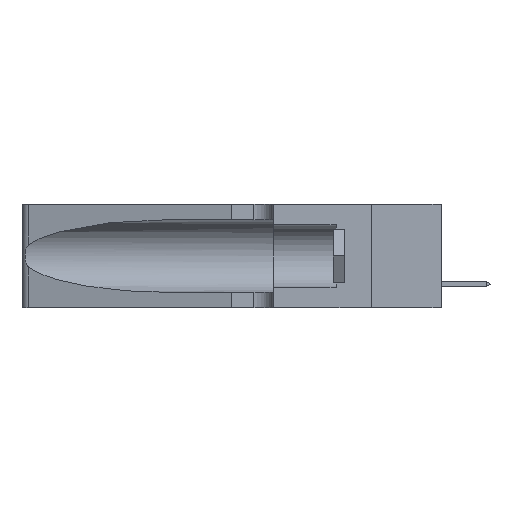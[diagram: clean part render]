
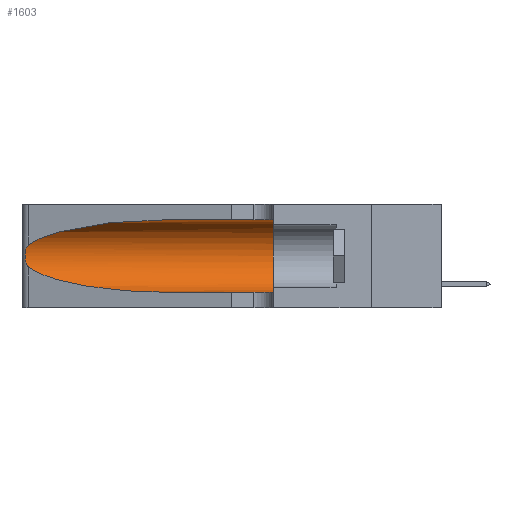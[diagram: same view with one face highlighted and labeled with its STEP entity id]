
A CAD part, left-side view. The second image highlights one B-rep face of the part: STEP entity #1603.
In plain terms, the highlighted cylindrical face has radius 3.308 mm (diameter 6.617 mm), a partial arc.
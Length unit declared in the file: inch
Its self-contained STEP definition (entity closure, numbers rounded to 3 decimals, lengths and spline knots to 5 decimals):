
#150 = AXIS2_PLACEMENT_3D ( 'NONE', #41424, #35982, #982 ) ;
#260 = VERTEX_POINT ( 'NONE', #41802 ) ;
#375 = EDGE_CURVE ( 'NONE', #417, #260, #31418, .T. ) ;
#417 = VERTEX_POINT ( 'NONE', #14140 ) ;
#982 = DIRECTION ( 'NONE',  ( 0., 0., 1. ) ) ;
#1032 = VERTEX_POINT ( 'NONE', #37937 ) ;
#1080 = VERTEX_POINT ( 'NONE', #20702 ) ;
#1603 = ADVANCED_FACE ( 'NONE', ( #44510 ), #25663, .F. ) ;
#2591 = CARTESIAN_POINT ( 'NONE',  ( 0.25555, 1.22993, 0.14849 ) ) ;
#4481 = EDGE_CURVE ( 'NONE', #1080, #30819, #5977, .T. ) ;
#5298 = VECTOR ( 'NONE', #27227, 39.37008 ) ;
#5703 = EDGE_CURVE ( 'NONE', #1080, #417, #10057, .T. ) ;
#5969 = CARTESIAN_POINT ( 'NONE',  ( 0.25487, 1.22718, 0.14631 ) ) ;
#5977 = LINE ( 'NONE', #21402, #46657 ) ;
#6178 = CARTESIAN_POINT ( 'NONE',  ( 0.25487, 1.22718, 0.14631 ) ) ;
#6469 = CARTESIAN_POINT ( 'NONE',  ( 0.25487, 1.22718, 0.22369 ) ) ;
#6504 = CARTESIAN_POINT ( 'NONE',  ( 0.26018, 1.23835, 0.19895 ) ) ;
#9677 = CARTESIAN_POINT ( 'NONE',  ( 0.25639, 1.23184, 0.21858 ) ) ;
#9921 = CIRCLE ( 'NONE', #150, 0.13025 ) ;
#9954 = CARTESIAN_POINT ( 'NONE',  ( 0.1305, 0.72297, 0.05475 ) ) ;
#9999 = CARTESIAN_POINT ( 'NONE',  ( 0.25639, 1.23186, 0.15144 ) ) ;
#10057 =( BOUNDED_CURVE ( )  B_SPLINE_CURVE ( 3, ( #39265, #17660, #21315, #6469 ),
 .UNSPECIFIED., .F., .F. ) 
 B_SPLINE_CURVE_WITH_KNOTS ( ( 4, 4 ),
 ( 1.5708, 2.84003 ),
 .UNSPECIFIED. ) 
 CURVE ( )  GEOMETRIC_REPRESENTATION_ITEM ( )  RATIONAL_B_SPLINE_CURVE ( ( 1., 0.87, 0.87, 1. ) ) 
 REPRESENTATION_ITEM ( '' )  );
#10159 = CARTESIAN_POINT ( 'NONE',  ( 0.26075, 1.23896, 0.178 ) ) ;
#11439 =( BOUNDED_CURVE ( )  B_SPLINE_CURVE ( 3, ( #5969, #35218, #43255, #9954 ),
 .UNSPECIFIED., .F., .F. ) 
 B_SPLINE_CURVE_WITH_KNOTS ( ( 4, 4 ),
 ( 3.44316, 4.71239 ),
 .UNSPECIFIED. ) 
 CURVE ( )  GEOMETRIC_REPRESENTATION_ITEM ( )  RATIONAL_B_SPLINE_CURVE ( ( 1., 0.87, 0.87, 1. ) ) 
 REPRESENTATION_ITEM ( '' )  );
#12462 = EDGE_LOOP ( 'NONE', ( #20390, #26127, #23223, #43813, #46731, #25531 ) ) ;
#13344 = CARTESIAN_POINT ( 'NONE',  ( 0.25854, 1.2359, 0.20912 ) ) ;
#14140 = CARTESIAN_POINT ( 'NONE',  ( 0.25487, 1.22718, 0.22369 ) ) ;
#14780 = EDGE_CURVE ( 'NONE', #31597, #1032, #15014, .T. ) ;
#15014 = LINE ( 'NONE', #30745, #5298 ) ;
#16245 = CARTESIAN_POINT ( 'NONE',  ( 0.1305, 0.72297, 0.05475 ) ) ;
#17043 = CARTESIAN_POINT ( 'NONE',  ( 0.25856, 1.23593, 0.16098 ) ) ;
#17660 = CARTESIAN_POINT ( 'NONE',  ( 0.18966, 0.96281, 0.31525 ) ) ;
#20390 = ORIENTED_EDGE ( 'NONE', *, *, #5703, .T. ) ;
#20414 = EDGE_CURVE ( 'NONE', #30819, #1032, #9921, .T. ) ;
#20702 = CARTESIAN_POINT ( 'NONE',  ( 0.1305, 0.72297, 0.31525 ) ) ;
#21315 = CARTESIAN_POINT ( 'NONE',  ( 0.2373, 1.15595, 0.28018 ) ) ;
#21402 = CARTESIAN_POINT ( 'NONE',  ( 0.1305, 1.61858, 0.31525 ) ) ;
#21856 = DIRECTION ( 'NONE',  ( 0., -1., 0. ) ) ;
#23223 = ORIENTED_EDGE ( 'NONE', *, *, #28506, .T. ) ;
#24023 = CARTESIAN_POINT ( 'NONE',  ( 0.1305, 1.61858, 0.185 ) ) ;
#24521 = CARTESIAN_POINT ( 'NONE',  ( 0.26017, 1.23833, 0.17102 ) ) ;
#25531 = ORIENTED_EDGE ( 'NONE', *, *, #4481, .F. ) ;
#25663 = CYLINDRICAL_SURFACE ( 'NONE', #47308, 0.13025 ) ;
#26127 = ORIENTED_EDGE ( 'NONE', *, *, #375, .T. ) ;
#26892 = CARTESIAN_POINT ( 'NONE',  ( 0.1305, 0.35, 0.31525 ) ) ;
#27227 = DIRECTION ( 'NONE',  ( 0., -1., 0. ) ) ;
#28053 = CARTESIAN_POINT ( 'NONE',  ( 0.25789, 1.23486, 0.15765 ) ) ;
#28395 = CARTESIAN_POINT ( 'NONE',  ( 0.25555, 1.22994, 0.2215 ) ) ;
#28506 = EDGE_CURVE ( 'NONE', #260, #31597, #11439, .T. ) ;
#30745 = CARTESIAN_POINT ( 'NONE',  ( 0.1305, 1.61858, 0.05475 ) ) ;
#30819 = VERTEX_POINT ( 'NONE', #26892 ) ;
#31418 = B_SPLINE_CURVE_WITH_KNOTS ( 'NONE', 3,
 ( #31581, #28395, #9677, #35261, #13344, #6504, #38979, #10159, #24521, #17043, #28053, #9999, #2591, #6178 ),
 .UNSPECIFIED., .F., .F.,
 ( 4, 2, 2, 2, 2, 2, 4 ),
 ( 0., 0.00027, 0.00053, 0.00107, 0.0016, 0.00187, 0.00214 ),
 .UNSPECIFIED. ) ;
#31581 = CARTESIAN_POINT ( 'NONE',  ( 0.25487, 1.22718, 0.22369 ) ) ;
#31597 = VERTEX_POINT ( 'NONE', #16245 ) ;
#35218 = CARTESIAN_POINT ( 'NONE',  ( 0.2373, 1.15595, 0.08982 ) ) ;
#35261 = CARTESIAN_POINT ( 'NONE',  ( 0.25787, 1.23484, 0.2124 ) ) ;
#35982 = DIRECTION ( 'NONE',  ( 0., 1., 0. ) ) ;
#37937 = CARTESIAN_POINT ( 'NONE',  ( 0.1305, 0.35, 0.05475 ) ) ;
#38145 = DIRECTION ( 'NONE',  ( 0., 0., -1. ) ) ;
#38316 = DIRECTION ( 'NONE',  ( 0., -1., 0. ) ) ;
#38979 = CARTESIAN_POINT ( 'NONE',  ( 0.26075, 1.23896, 0.19203 ) ) ;
#39265 = CARTESIAN_POINT ( 'NONE',  ( 0.1305, 0.72297, 0.31525 ) ) ;
#41424 = CARTESIAN_POINT ( 'NONE',  ( 0.1305, 0.35, 0.185 ) ) ;
#41802 = CARTESIAN_POINT ( 'NONE',  ( 0.25487, 1.22718, 0.14631 ) ) ;
#43255 = CARTESIAN_POINT ( 'NONE',  ( 0.18966, 0.96281, 0.05475 ) ) ;
#43813 = ORIENTED_EDGE ( 'NONE', *, *, #14780, .T. ) ;
#44510 = FACE_OUTER_BOUND ( 'NONE', #12462, .T. ) ;
#46657 = VECTOR ( 'NONE', #21856, 39.37008 ) ;
#46731 = ORIENTED_EDGE ( 'NONE', *, *, #20414, .F. ) ;
#47308 = AXIS2_PLACEMENT_3D ( 'NONE', #24023, #38316, #38145 ) ;
